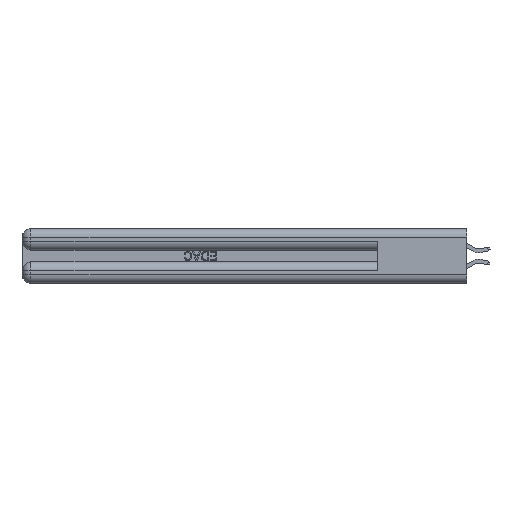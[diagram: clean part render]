
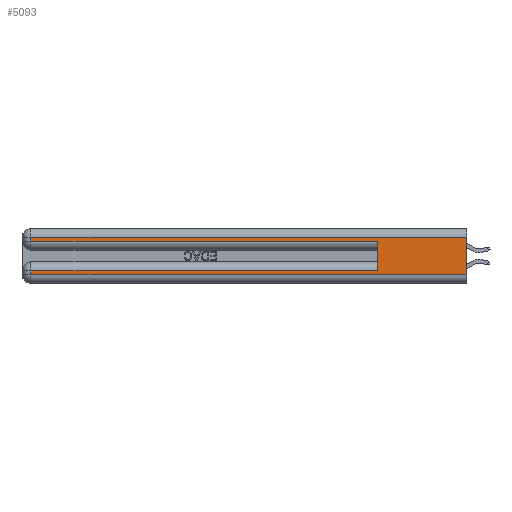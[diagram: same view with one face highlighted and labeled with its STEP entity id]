
A CAD part, left-side view. The second image highlights one B-rep face of the part: STEP entity #5093.
In plain terms, the highlighted planar face has unit normal (-1, 0, 0).
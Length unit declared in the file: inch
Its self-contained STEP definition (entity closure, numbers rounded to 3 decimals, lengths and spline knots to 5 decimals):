
#1720 = CARTESIAN_POINT ( 'NONE',  ( 0., 0., 0.37 ) ) ;
#2334 = DIRECTION ( 'NONE',  ( 0., 0., 1. ) ) ;
#2382 = VECTOR ( 'NONE', #10214, 39.37008 ) ;
#3643 = LINE ( 'NONE', #34078, #23462 ) ;
#3829 = VECTOR ( 'NONE', #27421, 39.37008 ) ;
#4093 = LINE ( 'NONE', #7093, #5287 ) ;
#5093 = ADVANCED_FACE ( 'NONE', ( #21616 ), #25157, .F. ) ;
#5287 = VECTOR ( 'NONE', #33097, 39.37008 ) ;
#5497 = DIRECTION ( 'NONE',  ( 0., 0., -1. ) ) ;
#6009 = DIRECTION ( 'NONE',  ( 0., 0., -1. ) ) ;
#6553 = VECTOR ( 'NONE', #6009, 39.37008 ) ;
#6615 = DIRECTION ( 'NONE',  ( 1., 0., 0. ) ) ;
#7093 = CARTESIAN_POINT ( 'NONE',  ( 0., 0., 0.285 ) ) ;
#8906 = EDGE_CURVE ( 'NONE', #24380, #34196, #20766, .T. ) ;
#10214 = DIRECTION ( 'NONE',  ( 0., -1., 0. ) ) ;
#11106 = EDGE_CURVE ( 'NONE', #20981, #44808, #21198, .T. ) ;
#11778 = ORIENTED_EDGE ( 'NONE', *, *, #44657, .T. ) ;
#11817 = DIRECTION ( 'NONE',  ( 0., 1., 0. ) ) ;
#12052 = EDGE_CURVE ( 'NONE', #20981, #41669, #29850, .T. ) ;
#13608 = CARTESIAN_POINT ( 'NONE',  ( 0., 0.6, 0.145 ) ) ;
#14821 = EDGE_CURVE ( 'NONE', #32965, #20979, #16425, .T. ) ;
#16065 = EDGE_LOOP ( 'NONE', ( #24185, #37356, #28383, #44712, #22119, #11778, #34372, #19262 ) ) ;
#16425 = LINE ( 'NONE', #17050, #6553 ) ;
#16745 = CARTESIAN_POINT ( 'NONE',  ( 0., 2.94, 0.31 ) ) ;
#17050 = CARTESIAN_POINT ( 'NONE',  ( 0., 2.94, 0.37 ) ) ;
#17653 = CARTESIAN_POINT ( 'NONE',  ( 0., 0., 0.37 ) ) ;
#19262 = ORIENTED_EDGE ( 'NONE', *, *, #45599, .T. ) ;
#19919 = CARTESIAN_POINT ( 'NONE',  ( 0., 0., 0.06 ) ) ;
#20766 = LINE ( 'NONE', #13608, #48033 ) ;
#20979 = VERTEX_POINT ( 'NONE', #21229 ) ;
#20981 = VERTEX_POINT ( 'NONE', #47190 ) ;
#21014 = CARTESIAN_POINT ( 'NONE',  ( 0., 0.6, 0.085 ) ) ;
#21015 = LINE ( 'NONE', #28772, #2382 ) ;
#21198 = LINE ( 'NONE', #1720, #22369 ) ;
#21229 = CARTESIAN_POINT ( 'NONE',  ( 0., 2.94, 0.06 ) ) ;
#21616 = FACE_OUTER_BOUND ( 'NONE', #16065, .T. ) ;
#22119 = ORIENTED_EDGE ( 'NONE', *, *, #8906, .F. ) ;
#22369 = VECTOR ( 'NONE', #5497, 39.37008 ) ;
#22378 = AXIS2_PLACEMENT_3D ( 'NONE', #17653, #6615, #32602 ) ;
#23462 = VECTOR ( 'NONE', #11817, 39.37008 ) ;
#23646 = LINE ( 'NONE', #34707, #3829 ) ;
#23865 = EDGE_CURVE ( 'NONE', #24912, #34196, #4093, .T. ) ;
#24185 = ORIENTED_EDGE ( 'NONE', *, *, #11106, .F. ) ;
#24380 = VERTEX_POINT ( 'NONE', #21014 ) ;
#24912 = VERTEX_POINT ( 'NONE', #48084 ) ;
#25157 = PLANE ( 'NONE',  #22378 ) ;
#25745 = DIRECTION ( 'NONE',  ( 0., 1., 0. ) ) ;
#27421 = DIRECTION ( 'NONE',  ( 0., 0., -1. ) ) ;
#28383 = ORIENTED_EDGE ( 'NONE', *, *, #42811, .T. ) ;
#28772 = CARTESIAN_POINT ( 'NONE',  ( 0., 0., 0.06 ) ) ;
#29850 = LINE ( 'NONE', #47922, #39708 ) ;
#32602 = DIRECTION ( 'NONE',  ( 0., 0., -1. ) ) ;
#32965 = VERTEX_POINT ( 'NONE', #34082 ) ;
#33097 = DIRECTION ( 'NONE',  ( 0., -1., 0. ) ) ;
#34078 = CARTESIAN_POINT ( 'NONE',  ( 0., 0., 0.085 ) ) ;
#34082 = CARTESIAN_POINT ( 'NONE',  ( 0., 2.94, 0.085 ) ) ;
#34196 = VERTEX_POINT ( 'NONE', #37743 ) ;
#34372 = ORIENTED_EDGE ( 'NONE', *, *, #14821, .T. ) ;
#34707 = CARTESIAN_POINT ( 'NONE',  ( 0., 2.94, 0.37 ) ) ;
#37356 = ORIENTED_EDGE ( 'NONE', *, *, #12052, .T. ) ;
#37743 = CARTESIAN_POINT ( 'NONE',  ( 0., 0.6, 0.285 ) ) ;
#39708 = VECTOR ( 'NONE', #25745, 39.37008 ) ;
#41669 = VERTEX_POINT ( 'NONE', #16745 ) ;
#42811 = EDGE_CURVE ( 'NONE', #41669, #24912, #23646, .T. ) ;
#44657 = EDGE_CURVE ( 'NONE', #24380, #32965, #3643, .T. ) ;
#44712 = ORIENTED_EDGE ( 'NONE', *, *, #23865, .T. ) ;
#44808 = VERTEX_POINT ( 'NONE', #19919 ) ;
#45599 = EDGE_CURVE ( 'NONE', #20979, #44808, #21015, .T. ) ;
#47190 = CARTESIAN_POINT ( 'NONE',  ( 0., 0., 0.31 ) ) ;
#47922 = CARTESIAN_POINT ( 'NONE',  ( 0., 0., 0.31 ) ) ;
#48033 = VECTOR ( 'NONE', #2334, 39.37008 ) ;
#48084 = CARTESIAN_POINT ( 'NONE',  ( 0., 2.94, 0.285 ) ) ;
